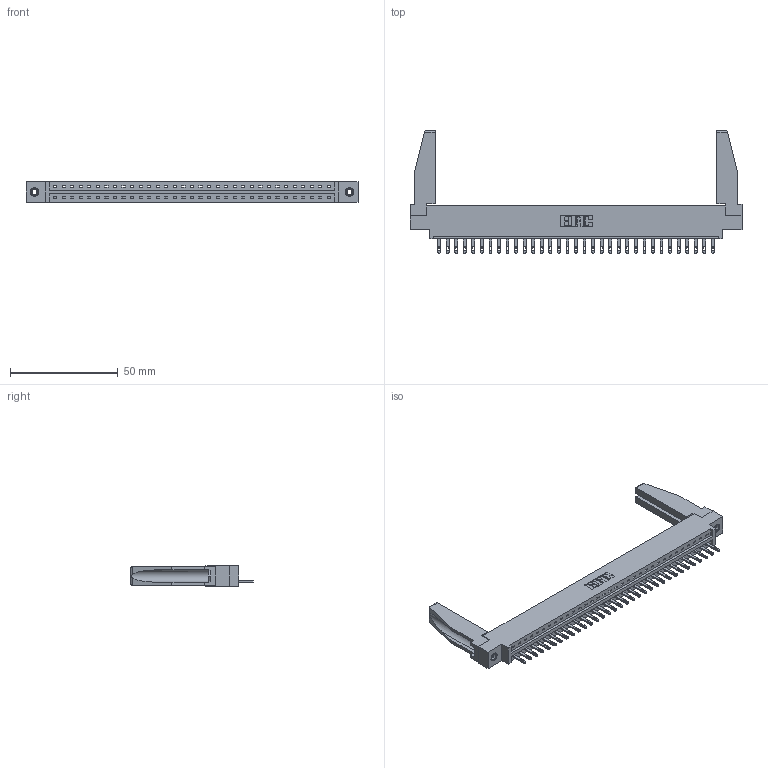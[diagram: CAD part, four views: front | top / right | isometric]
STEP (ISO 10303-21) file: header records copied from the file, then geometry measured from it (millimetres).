
FILE_DESCRIPTION (( 'STEP AP203' ), '1' );
FILE_NAME ('337-033-500-678.STEP', '2019-10-01T04:04:21', ( '' ), ( '' ), 'SwSTEP 2.0', 'SolidWorks 2016', '' );
FILE_SCHEMA (( 'CONFIG_CONTROL_DESIGN' ));
Length unit declared in the file: inch
Products named in the file (5): 337 Part_0.170 Offset - 0.156 Dia-TI; 337-033-500-678; 345-292-001_345-293-100; 307-220-078; 345-250-001_345-250-001-102
Assembly tree (38 placements, depth 2):
  337-033-500-678
    337 Part_0.170 Offset - 0.156 Dia-TI
    345-292-001_345-293-100  x33
    345-250-001_345-250-001-102  x2
    307-220-078  x2
Bounding box: 153.77 x 56.65 x 9.4 mm (x, y, z)
Volume: 19765.6 mm3; surface area: 20258.7 mm2
Topology: 38 solids, 38 shells, 2162 faces, 6593 edges, 4386 vertices
Faces by surface type: plane 1478, cylinder 668, cone 12, torus 4
Entity records: 28196 total; most frequent: CARTESIAN_POINT 4903, ORIENTED_EDGE 4828, DIRECTION 4156, EDGE_CURVE 2414, LINE 2244, VECTOR 2244, VERTEX_POINT 1604, AXIS2_PLACEMENT_3D 956
